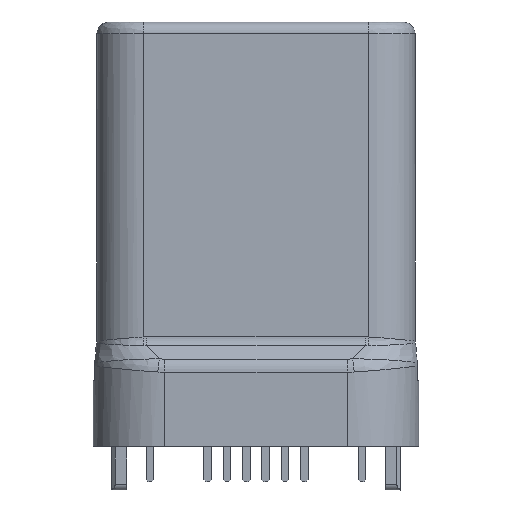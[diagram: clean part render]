
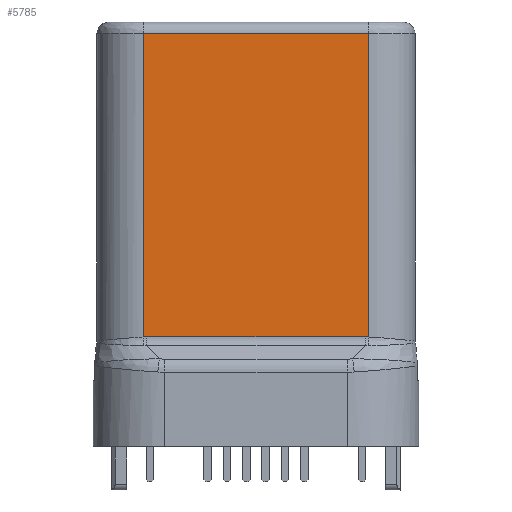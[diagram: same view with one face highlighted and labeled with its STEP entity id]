
A CAD part, front view. The second image highlights one B-rep face of the part: STEP entity #5785.
In plain terms, the highlighted planar face has unit normal (0, -1, 0).
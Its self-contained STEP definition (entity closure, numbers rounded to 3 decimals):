
#1340 = ORIENTED_EDGE ( 'NONE', *, *, #45470, .T. ) ;
#1628 = CARTESIAN_POINT ( 'NONE',  ( 0., -1.2, -4.05 ) ) ;
#3019 = ORIENTED_EDGE ( 'NONE', *, *, #22071, .T. ) ;
#5298 = CARTESIAN_POINT ( 'NONE',  ( 2.925, -1.2, -4.05 ) ) ;
#5601 = LINE ( 'NONE', #5298, #28695 ) ;
#5785 = ADVANCED_FACE ( 'NONE', ( #18680 ), #40536, .T. ) ;
#10797 = VECTOR ( 'NONE', #40204, 1000. ) ;
#12172 = CARTESIAN_POINT ( 'NONE',  ( -2.925, -1.2, -0.2 ) ) ;
#13548 = DIRECTION ( 'NONE',  ( 0., 0., 1. ) ) ;
#14351 = CARTESIAN_POINT ( 'NONE',  ( -2.925, -1.2, -4.05 ) ) ;
#14354 = VERTEX_POINT ( 'NONE', #38310 ) ;
#14972 = LINE ( 'NONE', #15256, #53292 ) ;
#15157 = EDGE_CURVE ( 'NONE', #50239, #14354, #38452, .T. ) ;
#15256 = CARTESIAN_POINT ( 'NONE',  ( 0., -1.2, -0.2 ) ) ;
#15404 = CARTESIAN_POINT ( 'NONE',  ( -2.838, -1.2, -8.063 ) ) ;
#18680 = FACE_OUTER_BOUND ( 'NONE', #50036, .T. ) ;
#18961 = DIRECTION ( 'NONE',  ( 0., -1., 0. ) ) ;
#21989 = EDGE_CURVE ( 'NONE', #52005, #27259, #32944, .T. ) ;
#22071 = EDGE_CURVE ( 'NONE', #27259, #50239, #34329, .T. ) ;
#22325 = DIRECTION ( 'NONE',  ( 1., 0., 0. ) ) ;
#22355 = VECTOR ( 'NONE', #42167, 1000. ) ;
#27259 = VERTEX_POINT ( 'NONE', #15404 ) ;
#28127 = CARTESIAN_POINT ( 'NONE',  ( -2.925, -1.2, -8.065 ) ) ;
#28695 = VECTOR ( 'NONE', #13548, 1000. ) ;
#32617 = VECTOR ( 'NONE', #22325, 1000. ) ;
#32944 = LINE ( 'NONE', #28127, #56162 ) ;
#32955 = CARTESIAN_POINT ( 'NONE',  ( -2.925, -1.2, -8.065 ) ) ;
#33876 = VERTEX_POINT ( 'NONE', #12172 ) ;
#34084 = ORIENTED_EDGE ( 'NONE', *, *, #21989, .T. ) ;
#34329 = LINE ( 'NONE', #51689, #32617 ) ;
#34528 = ORIENTED_EDGE ( 'NONE', *, *, #15157, .T. ) ;
#34762 = CARTESIAN_POINT ( 'NONE',  ( 2.838, -1.2, -8.063 ) ) ;
#35026 = ORIENTED_EDGE ( 'NONE', *, *, #47976, .T. ) ;
#36215 = LINE ( 'NONE', #14351, #10797 ) ;
#38310 = CARTESIAN_POINT ( 'NONE',  ( 2.925, -1.2, -8.065 ) ) ;
#38452 = LINE ( 'NONE', #55274, #22355 ) ;
#40204 = DIRECTION ( 'NONE',  ( 0., 0., -1. ) ) ;
#40536 = PLANE ( 'NONE',  #42501 ) ;
#42167 = DIRECTION ( 'NONE',  ( 1., 0., -0.025 ) ) ;
#42501 = AXIS2_PLACEMENT_3D ( 'NONE', #1628, #18961, #49930 ) ;
#43309 = VERTEX_POINT ( 'NONE', #50879 ) ;
#44622 = ORIENTED_EDGE ( 'NONE', *, *, #50615, .T. ) ;
#45470 = EDGE_CURVE ( 'NONE', #33876, #52005, #36215, .T. ) ;
#47976 = EDGE_CURVE ( 'NONE', #14354, #43309, #5601, .T. ) ;
#49930 = DIRECTION ( 'NONE',  ( 0., 0., -1. ) ) ;
#50036 = EDGE_LOOP ( 'NONE', ( #44622, #1340, #34084, #3019, #34528, #35026 ) ) ;
#50239 = VERTEX_POINT ( 'NONE', #34762 ) ;
#50615 = EDGE_CURVE ( 'NONE', #43309, #33876, #14972, .T. ) ;
#50879 = CARTESIAN_POINT ( 'NONE',  ( 2.925, -1.2, -0.2 ) ) ;
#51689 = CARTESIAN_POINT ( 'NONE',  ( 0., -1.2, -8.063 ) ) ;
#52005 = VERTEX_POINT ( 'NONE', #32955 ) ;
#53292 = VECTOR ( 'NONE', #53945, 1000. ) ;
#53945 = DIRECTION ( 'NONE',  ( -1., 0., 0. ) ) ;
#54583 = DIRECTION ( 'NONE',  ( 1., 0., 0.025 ) ) ;
#55274 = CARTESIAN_POINT ( 'NONE',  ( 2.838, -1.2, -8.063 ) ) ;
#56162 = VECTOR ( 'NONE', #54583, 1000. ) ;
